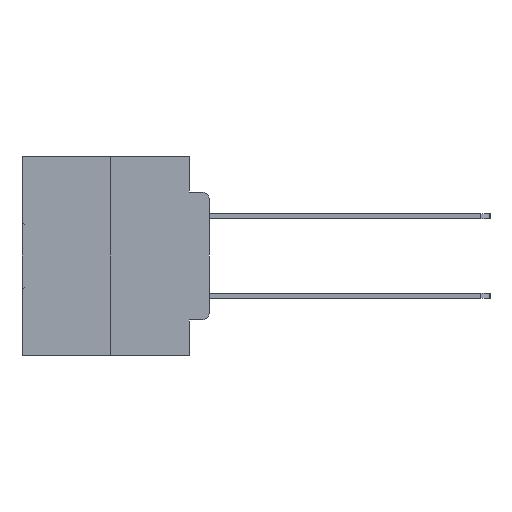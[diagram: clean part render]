
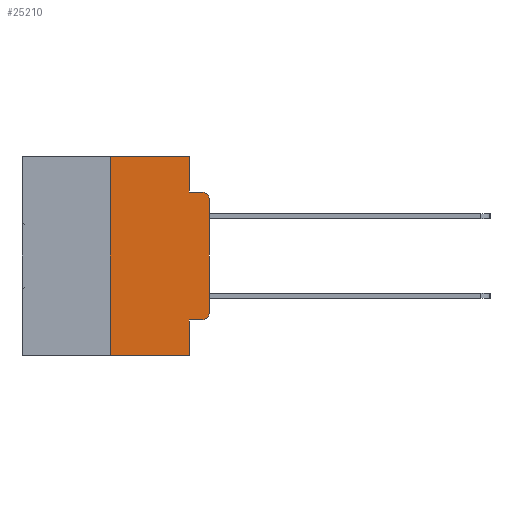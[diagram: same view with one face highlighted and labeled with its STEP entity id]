
A CAD part, left-side view. The second image highlights one B-rep face of the part: STEP entity #25210.
In plain terms, the highlighted planar face has unit normal (-1, 0, 0).
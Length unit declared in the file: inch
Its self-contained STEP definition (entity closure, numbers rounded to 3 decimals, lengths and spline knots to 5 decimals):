
#549 = VERTEX_POINT ( 'NONE', #3589 ) ;
#583 = EDGE_CURVE ( 'NONE', #3791, #24227, #5342, .T. ) ;
#744 = DIRECTION ( 'NONE',  ( 1., 0., 0. ) ) ;
#1283 = LINE ( 'NONE', #22202, #20423 ) ;
#2450 = CARTESIAN_POINT ( 'NONE',  ( 0., 0.473, -0.5 ) ) ;
#2488 = CARTESIAN_POINT ( 'NONE',  ( 0., 0.051, -0.5 ) ) ;
#3306 = VERTEX_POINT ( 'NONE', #12912 ) ;
#3342 = CARTESIAN_POINT ( 'NONE',  ( 0., 0.25, -0.5 ) ) ;
#3589 = CARTESIAN_POINT ( 'NONE',  ( 0., 0.051, -0.4115 ) ) ;
#3681 = DIRECTION ( 'NONE',  ( 0., 0., 1. ) ) ;
#3791 = VERTEX_POINT ( 'NONE', #3342 ) ;
#3847 = ORIENTED_EDGE ( 'NONE', *, *, #583, .F. ) ;
#4156 = EDGE_CURVE ( 'NONE', #3791, #13164, #28271, .T. ) ;
#4181 = CARTESIAN_POINT ( 'NONE',  ( 0., 0.051, -0.0885 ) ) ;
#4268 = CARTESIAN_POINT ( 'NONE',  ( 0., 0.02, -0.3915 ) ) ;
#4860 = ORIENTED_EDGE ( 'NONE', *, *, #24918, .T. ) ;
#5342 = LINE ( 'NONE', #26043, #11186 ) ;
#5369 = ORIENTED_EDGE ( 'NONE', *, *, #28096, .T. ) ;
#6575 = CARTESIAN_POINT ( 'NONE',  ( 0., 0., -0.1085 ) ) ;
#6792 = DIRECTION ( 'NONE',  ( 0., 0., -1. ) ) ;
#6807 = VECTOR ( 'NONE', #9604, 39.37008 ) ;
#7106 = CARTESIAN_POINT ( 'NONE',  ( 0., 0.051, -0.4115 ) ) ;
#9441 = VERTEX_POINT ( 'NONE', #23333 ) ;
#9451 = AXIS2_PLACEMENT_3D ( 'NONE', #13182, #744, #18200 ) ;
#9604 = DIRECTION ( 'NONE',  ( 0., -1., 0. ) ) ;
#10121 = DIRECTION ( 'NONE',  ( -1., 0., 0. ) ) ;
#11186 = VECTOR ( 'NONE', #3681, 39.37008 ) ;
#11276 = VERTEX_POINT ( 'NONE', #27168 ) ;
#11856 = EDGE_LOOP ( 'NONE', ( #28764, #5369, #28236, #25416, #13235, #3847, #31904, #21634, #4860, #31685 ) ) ;
#12912 = CARTESIAN_POINT ( 'NONE',  ( 0., 0., -0.3915 ) ) ;
#13164 = VERTEX_POINT ( 'NONE', #2488 ) ;
#13182 = CARTESIAN_POINT ( 'NONE',  ( 0., 0.473, 0. ) ) ;
#13235 = ORIENTED_EDGE ( 'NONE', *, *, #22595, .F. ) ;
#14070 = AXIS2_PLACEMENT_3D ( 'NONE', #4268, #21703, #6792 ) ;
#14365 = LINE ( 'NONE', #18759, #26846 ) ;
#14688 = DIRECTION ( 'NONE',  ( 0., 0., -1. ) ) ;
#14789 = LINE ( 'NONE', #20508, #31538 ) ;
#15029 = VECTOR ( 'NONE', #32313, 39.37008 ) ;
#15285 = CARTESIAN_POINT ( 'NONE',  ( 0., 0.25, 0. ) ) ;
#17263 = VECTOR ( 'NONE', #20928, 39.37008 ) ;
#17565 = EDGE_CURVE ( 'NONE', #549, #13164, #31279, .T. ) ;
#18115 = CARTESIAN_POINT ( 'NONE',  ( 0., 0.02, -0.0885 ) ) ;
#18200 = DIRECTION ( 'NONE',  ( 0., 0., -1. ) ) ;
#18759 = CARTESIAN_POINT ( 'NONE',  ( 0., 0.473, 0. ) ) ;
#19679 = FACE_OUTER_BOUND ( 'NONE', #11856, .T. ) ;
#19915 = CARTESIAN_POINT ( 'NONE',  ( 0., 0.051, -0.0885 ) ) ;
#20423 = VECTOR ( 'NONE', #14688, 39.37008 ) ;
#20508 = CARTESIAN_POINT ( 'NONE',  ( 0., 0., 0. ) ) ;
#20928 = DIRECTION ( 'NONE',  ( 0., 0., -1. ) ) ;
#21228 = DIRECTION ( 'NONE',  ( 0., -1., 0. ) ) ;
#21439 = VERTEX_POINT ( 'NONE', #4181 ) ;
#21594 = EDGE_CURVE ( 'NONE', #21439, #22441, #23391, .T. ) ;
#21634 = ORIENTED_EDGE ( 'NONE', *, *, #17565, .F. ) ;
#21703 = DIRECTION ( 'NONE',  ( -1., 0., 0. ) ) ;
#22187 = DIRECTION ( 'NONE',  ( 0., -1., 0. ) ) ;
#22202 = CARTESIAN_POINT ( 'NONE',  ( 0., 0.051, 0. ) ) ;
#22414 = EDGE_CURVE ( 'NONE', #3306, #26143, #14789, .T. ) ;
#22441 = VERTEX_POINT ( 'NONE', #18115 ) ;
#22595 = EDGE_CURVE ( 'NONE', #24227, #11276, #14365, .T. ) ;
#22617 = VECTOR ( 'NONE', #22187, 39.37008 ) ;
#23333 = CARTESIAN_POINT ( 'NONE',  ( 0., 0.02, -0.4115 ) ) ;
#23335 = CARTESIAN_POINT ( 'NONE',  ( 0., 0.051, 0. ) ) ;
#23391 = LINE ( 'NONE', #19915, #22617 ) ;
#24227 = VERTEX_POINT ( 'NONE', #15285 ) ;
#24918 = EDGE_CURVE ( 'NONE', #549, #9441, #26698, .T. ) ;
#25071 = CARTESIAN_POINT ( 'NONE',  ( 0., 0.02, -0.1085 ) ) ;
#25210 = ADVANCED_FACE ( 'NONE', ( #19679 ), #30619, .F. ) ;
#25416 = ORIENTED_EDGE ( 'NONE', *, *, #25622, .F. ) ;
#25622 = EDGE_CURVE ( 'NONE', #11276, #21439, #1283, .T. ) ;
#26043 = CARTESIAN_POINT ( 'NONE',  ( 0., 0.25, 0. ) ) ;
#26143 = VERTEX_POINT ( 'NONE', #6575 ) ;
#26698 = LINE ( 'NONE', #7106, #6807 ) ;
#26846 = VECTOR ( 'NONE', #21228, 39.37008 ) ;
#27168 = CARTESIAN_POINT ( 'NONE',  ( 0., 0.051, 0. ) ) ;
#27235 = EDGE_CURVE ( 'NONE', #9441, #3306, #30439, .T. ) ;
#27559 = DIRECTION ( 'NONE',  ( 0., 0., -1. ) ) ;
#28096 = EDGE_CURVE ( 'NONE', #26143, #22441, #31935, .T. ) ;
#28236 = ORIENTED_EDGE ( 'NONE', *, *, #21594, .F. ) ;
#28271 = LINE ( 'NONE', #2450, #15029 ) ;
#28764 = ORIENTED_EDGE ( 'NONE', *, *, #22414, .T. ) ;
#29360 = AXIS2_PLACEMENT_3D ( 'NONE', #25071, #10121, #27559 ) ;
#30439 = CIRCLE ( 'NONE', #14070, 0.02 ) ;
#30534 = DIRECTION ( 'NONE',  ( 0., 0., 1. ) ) ;
#30619 = PLANE ( 'NONE',  #9451 ) ;
#31279 = LINE ( 'NONE', #23335, #17263 ) ;
#31538 = VECTOR ( 'NONE', #30534, 39.37008 ) ;
#31685 = ORIENTED_EDGE ( 'NONE', *, *, #27235, .T. ) ;
#31904 = ORIENTED_EDGE ( 'NONE', *, *, #4156, .T. ) ;
#31935 = CIRCLE ( 'NONE', #29360, 0.02 ) ;
#32313 = DIRECTION ( 'NONE',  ( 0., -1., 0. ) ) ;
